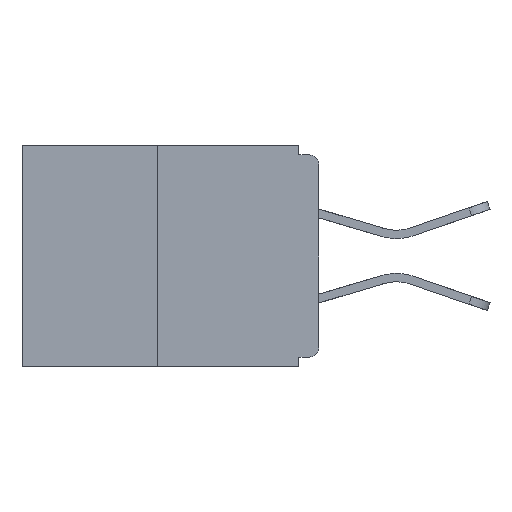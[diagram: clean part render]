
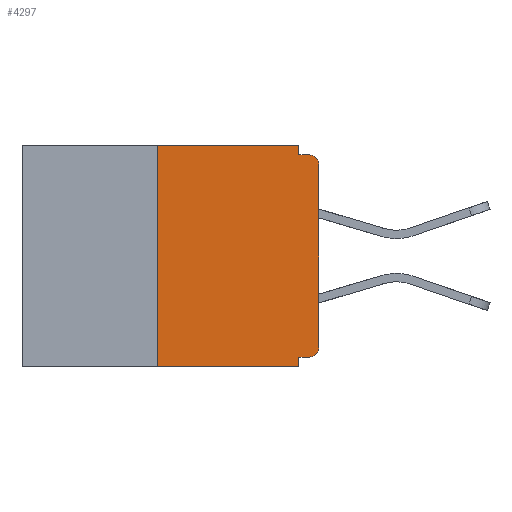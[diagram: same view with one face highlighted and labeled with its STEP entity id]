
A CAD part, left-side view. The second image highlights one B-rep face of the part: STEP entity #4297.
In plain terms, the highlighted planar face has unit normal (-1, 0, 0).
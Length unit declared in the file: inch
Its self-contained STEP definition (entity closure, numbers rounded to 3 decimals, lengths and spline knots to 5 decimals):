
#323 = ORIENTED_EDGE ( 'NONE', *, *, #13392, .F. ) ;
#1033 = VERTEX_POINT ( 'NONE', #17532 ) ;
#1055 = VERTEX_POINT ( 'NONE', #15777 ) ;
#1441 = CARTESIAN_POINT ( 'NONE',  ( 0., 0.031, -0.015 ) ) ;
#1625 = EDGE_LOOP ( 'NONE', ( #5963, #19347, #21358, #5245, #323, #9284, #9029, #10192, #2244, #2090 ) ) ;
#1647 = LINE ( 'NONE', #5106, #10472 ) ;
#1748 = FACE_OUTER_BOUND ( 'NONE', #1625, .T. ) ;
#1907 = DIRECTION ( 'NONE',  ( 0., -1., 0. ) ) ;
#2090 = ORIENTED_EDGE ( 'NONE', *, *, #10524, .F. ) ;
#2244 = ORIENTED_EDGE ( 'NONE', *, *, #16434, .F. ) ;
#2734 = DIRECTION ( 'NONE',  ( 0., 0., -1. ) ) ;
#3084 = LINE ( 'NONE', #11956, #4653 ) ;
#3190 = DIRECTION ( 'NONE',  ( 0., 0., 1. ) ) ;
#3429 = EDGE_CURVE ( 'NONE', #5833, #1033, #15327, .T. ) ;
#3734 = CARTESIAN_POINT ( 'NONE',  ( 0., 0.25, 0. ) ) ;
#4201 = CARTESIAN_POINT ( 'NONE',  ( 0., 0.015, -0.313 ) ) ;
#4297 = ADVANCED_FACE ( 'NONE', ( #1748 ), #4448, .F. ) ;
#4367 = AXIS2_PLACEMENT_3D ( 'NONE', #12572, #7646, #2734 ) ;
#4448 = PLANE ( 'NONE',  #8192 ) ;
#4653 = VECTOR ( 'NONE', #16848, 39.37008 ) ;
#5106 = CARTESIAN_POINT ( 'NONE',  ( 0., 0.46, 0. ) ) ;
#5245 = ORIENTED_EDGE ( 'NONE', *, *, #19409, .F. ) ;
#5809 = EDGE_CURVE ( 'NONE', #17671, #15767, #16767, .T. ) ;
#5833 = VERTEX_POINT ( 'NONE', #14377 ) ;
#5919 = DIRECTION ( 'NONE',  ( -1., 0., 0. ) ) ;
#5963 = ORIENTED_EDGE ( 'NONE', *, *, #20194, .F. ) ;
#6412 = AXIS2_PLACEMENT_3D ( 'NONE', #4201, #5919, #17406 ) ;
#6601 = VERTEX_POINT ( 'NONE', #8627 ) ;
#6603 = VECTOR ( 'NONE', #12182, 39.37008 ) ;
#6663 = DIRECTION ( 'NONE',  ( 0., -1., 0. ) ) ;
#6972 = EDGE_CURVE ( 'NONE', #20751, #1055, #9962, .T. ) ;
#7008 = LINE ( 'NONE', #13276, #9871 ) ;
#7646 = DIRECTION ( 'NONE',  ( -1., 0., 0. ) ) ;
#7806 = CARTESIAN_POINT ( 'NONE',  ( 0., 0.46, -0.343 ) ) ;
#8192 = AXIS2_PLACEMENT_3D ( 'NONE', #20974, #12710, #16067 ) ;
#8401 = DIRECTION ( 'NONE',  ( 0., 0., 1. ) ) ;
#8627 = CARTESIAN_POINT ( 'NONE',  ( 0., 0.25, 0. ) ) ;
#8697 = DIRECTION ( 'NONE',  ( 0., 0., -1. ) ) ;
#8954 = CARTESIAN_POINT ( 'NONE',  ( 0., 0.031, -0.328 ) ) ;
#9029 = ORIENTED_EDGE ( 'NONE', *, *, #16786, .T. ) ;
#9284 = ORIENTED_EDGE ( 'NONE', *, *, #3429, .T. ) ;
#9729 = LINE ( 'NONE', #18684, #6603 ) ;
#9871 = VECTOR ( 'NONE', #18496, 39.37008 ) ;
#9962 = LINE ( 'NONE', #7806, #13900 ) ;
#10192 = ORIENTED_EDGE ( 'NONE', *, *, #5809, .T. ) ;
#10472 = VECTOR ( 'NONE', #1907, 39.37008 ) ;
#10524 = EDGE_CURVE ( 'NONE', #14235, #16836, #13162, .T. ) ;
#10597 = CARTESIAN_POINT ( 'NONE',  ( 0., 0.25, -0.343 ) ) ;
#11956 = CARTESIAN_POINT ( 'NONE',  ( 0., 0., -0.015 ) ) ;
#12088 = VECTOR ( 'NONE', #8697, 39.37008 ) ;
#12182 = DIRECTION ( 'NONE',  ( 0., 0., -1. ) ) ;
#12572 = CARTESIAN_POINT ( 'NONE',  ( 0., 0.015, -0.03 ) ) ;
#12710 = DIRECTION ( 'NONE',  ( 1., 0., 0. ) ) ;
#12993 = CARTESIAN_POINT ( 'NONE',  ( 0., 0., 0. ) ) ;
#13162 = LINE ( 'NONE', #13666, #12088 ) ;
#13276 = CARTESIAN_POINT ( 'NONE',  ( 0., 0., -0.328 ) ) ;
#13392 = EDGE_CURVE ( 'NONE', #5833, #21012, #7008, .T. ) ;
#13666 = CARTESIAN_POINT ( 'NONE',  ( 0., 0.031, 0. ) ) ;
#13900 = VECTOR ( 'NONE', #6663, 39.37008 ) ;
#14235 = VERTEX_POINT ( 'NONE', #14329 ) ;
#14329 = CARTESIAN_POINT ( 'NONE',  ( 0., 0.031, 0. ) ) ;
#14377 = CARTESIAN_POINT ( 'NONE',  ( 0., 0.015, -0.328 ) ) ;
#15027 = LINE ( 'NONE', #12993, #18394 ) ;
#15327 = CIRCLE ( 'NONE', #6412, 0.015 ) ;
#15665 = VECTOR ( 'NONE', #8401, 39.37008 ) ;
#15767 = VERTEX_POINT ( 'NONE', #19083 ) ;
#15777 = CARTESIAN_POINT ( 'NONE',  ( 0., 0.031, -0.343 ) ) ;
#16067 = DIRECTION ( 'NONE',  ( 0., 0., -1. ) ) ;
#16434 = EDGE_CURVE ( 'NONE', #16836, #15767, #3084, .T. ) ;
#16767 = CIRCLE ( 'NONE', #4367, 0.015 ) ;
#16786 = EDGE_CURVE ( 'NONE', #1033, #17671, #15027, .T. ) ;
#16836 = VERTEX_POINT ( 'NONE', #1441 ) ;
#16848 = DIRECTION ( 'NONE',  ( 0., -1., 0. ) ) ;
#17406 = DIRECTION ( 'NONE',  ( 0., 0., -1. ) ) ;
#17532 = CARTESIAN_POINT ( 'NONE',  ( 0., 0., -0.313 ) ) ;
#17671 = VERTEX_POINT ( 'NONE', #18156 ) ;
#18156 = CARTESIAN_POINT ( 'NONE',  ( 0., 0., -0.03 ) ) ;
#18394 = VECTOR ( 'NONE', #3190, 39.37008 ) ;
#18496 = DIRECTION ( 'NONE',  ( 0., 1., 0. ) ) ;
#18684 = CARTESIAN_POINT ( 'NONE',  ( 0., 0.031, -0.343 ) ) ;
#19083 = CARTESIAN_POINT ( 'NONE',  ( 0., 0.015, -0.015 ) ) ;
#19347 = ORIENTED_EDGE ( 'NONE', *, *, #20164, .F. ) ;
#19409 = EDGE_CURVE ( 'NONE', #21012, #1055, #9729, .T. ) ;
#19614 = LINE ( 'NONE', #3734, #15665 ) ;
#20164 = EDGE_CURVE ( 'NONE', #20751, #6601, #19614, .T. ) ;
#20194 = EDGE_CURVE ( 'NONE', #6601, #14235, #1647, .T. ) ;
#20751 = VERTEX_POINT ( 'NONE', #10597 ) ;
#20974 = CARTESIAN_POINT ( 'NONE',  ( 0., 0.46, 0. ) ) ;
#21012 = VERTEX_POINT ( 'NONE', #8954 ) ;
#21358 = ORIENTED_EDGE ( 'NONE', *, *, #6972, .T. ) ;
